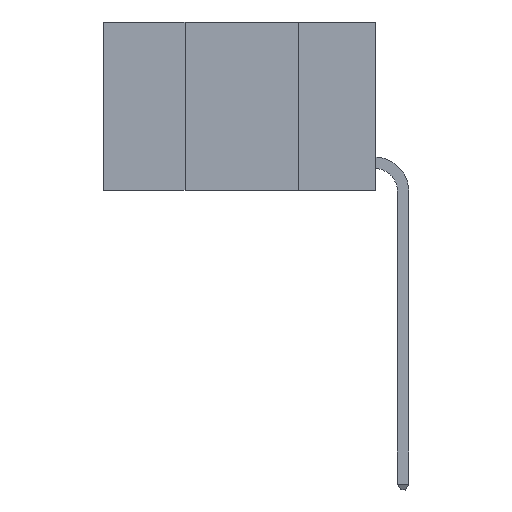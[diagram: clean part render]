
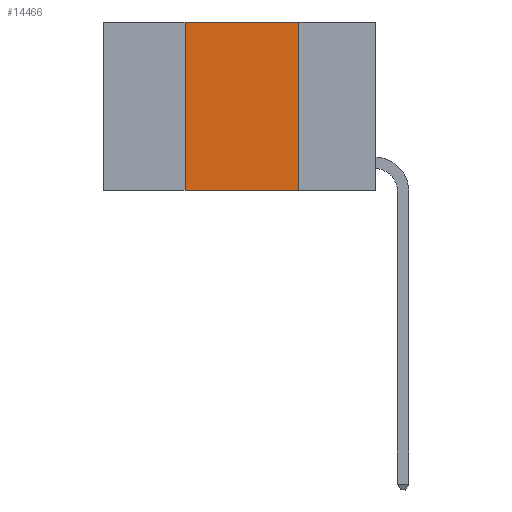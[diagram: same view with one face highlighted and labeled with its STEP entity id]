
A CAD part, left-side view. The second image highlights one B-rep face of the part: STEP entity #14466.
In plain terms, the highlighted planar face has unit normal (-1, 0, 0).
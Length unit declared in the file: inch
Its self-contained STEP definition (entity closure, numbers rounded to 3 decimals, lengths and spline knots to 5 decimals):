
#164 = DIRECTION ( 'NONE',  ( 0., 0., 1. ) ) ;
#994 = DIRECTION ( 'NONE',  ( 0., 0., -1. ) ) ;
#2877 = CARTESIAN_POINT ( 'NONE',  ( 0., 0.17, 0. ) ) ;
#3112 = DIRECTION ( 'NONE',  ( 0., -1., 0. ) ) ;
#3711 = VECTOR ( 'NONE', #3112, 39.37008 ) ;
#5258 = CARTESIAN_POINT ( 'NONE',  ( 0., 0.42, -0.37 ) ) ;
#6585 = ORIENTED_EDGE ( 'NONE', *, *, #9723, .F. ) ;
#7819 = VERTEX_POINT ( 'NONE', #2877 ) ;
#8602 = DIRECTION ( 'NONE',  ( 1., 0., 0. ) ) ;
#8924 = CARTESIAN_POINT ( 'NONE',  ( 0., 0.42, 0. ) ) ;
#9603 = LINE ( 'NONE', #27334, #20614 ) ;
#9723 = EDGE_CURVE ( 'NONE', #24627, #15787, #11548, .T. ) ;
#10694 = CARTESIAN_POINT ( 'NONE',  ( 0., 0.6, 0. ) ) ;
#11073 = FACE_OUTER_BOUND ( 'NONE', #14993, .T. ) ;
#11548 = LINE ( 'NONE', #8924, #21892 ) ;
#12650 = ORIENTED_EDGE ( 'NONE', *, *, #20433, .F. ) ;
#14190 = DIRECTION ( 'NONE',  ( 0., -1., 0. ) ) ;
#14466 = ADVANCED_FACE ( 'NONE', ( #11073 ), #21774, .F. ) ;
#14852 = VECTOR ( 'NONE', #994, 39.37008 ) ;
#14993 = EDGE_LOOP ( 'NONE', ( #12650, #22992, #6585, #20512 ) ) ;
#15787 = VERTEX_POINT ( 'NONE', #16461 ) ;
#16239 = LINE ( 'NONE', #16312, #14852 ) ;
#16312 = CARTESIAN_POINT ( 'NONE',  ( 0., 0.17, 0. ) ) ;
#16461 = CARTESIAN_POINT ( 'NONE',  ( 0., 0.42, 0. ) ) ;
#19949 = AXIS2_PLACEMENT_3D ( 'NONE', #10694, #8602, #23944 ) ;
#20433 = EDGE_CURVE ( 'NONE', #7819, #21926, #16239, .T. ) ;
#20512 = ORIENTED_EDGE ( 'NONE', *, *, #27238, .T. ) ;
#20614 = VECTOR ( 'NONE', #14190, 39.37008 ) ;
#21774 = PLANE ( 'NONE',  #19949 ) ;
#21892 = VECTOR ( 'NONE', #164, 39.37008 ) ;
#21926 = VERTEX_POINT ( 'NONE', #23856 ) ;
#22841 = CARTESIAN_POINT ( 'NONE',  ( 0., 0.6, -0.37 ) ) ;
#22992 = ORIENTED_EDGE ( 'NONE', *, *, #27269, .F. ) ;
#23856 = CARTESIAN_POINT ( 'NONE',  ( 0., 0.17, -0.37 ) ) ;
#23944 = DIRECTION ( 'NONE',  ( 0., 0., -1. ) ) ;
#24627 = VERTEX_POINT ( 'NONE', #5258 ) ;
#27098 = LINE ( 'NONE', #22841, #3711 ) ;
#27238 = EDGE_CURVE ( 'NONE', #24627, #21926, #27098, .T. ) ;
#27269 = EDGE_CURVE ( 'NONE', #15787, #7819, #9603, .T. ) ;
#27334 = CARTESIAN_POINT ( 'NONE',  ( 0., 0.6, 0. ) ) ;
